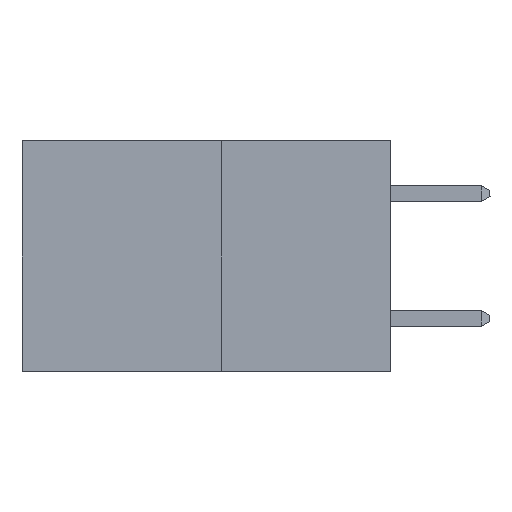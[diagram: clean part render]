
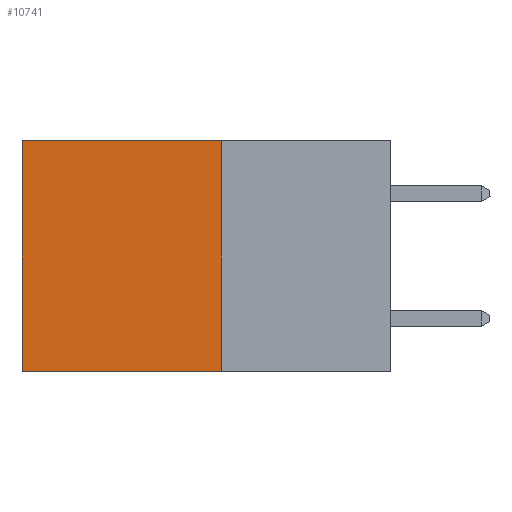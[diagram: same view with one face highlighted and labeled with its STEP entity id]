
A CAD part, left-side view. The second image highlights one B-rep face of the part: STEP entity #10741.
In plain terms, the highlighted planar face has unit normal (-1, 0, 0).
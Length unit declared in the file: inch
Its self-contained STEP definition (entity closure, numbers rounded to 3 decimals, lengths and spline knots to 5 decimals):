
#1203 = VERTEX_POINT ( 'NONE', #9209 ) ;
#1303 = DIRECTION ( 'NONE',  ( 0., 0., -1. ) ) ;
#1723 = VERTEX_POINT ( 'NONE', #7857 ) ;
#1883 = ORIENTED_EDGE ( 'NONE', *, *, #22564, .T. ) ;
#1886 = CARTESIAN_POINT ( 'NONE',  ( 0.277, 0.27, -0.37 ) ) ;
#2969 = EDGE_CURVE ( 'NONE', #15970, #17528, #15374, .T. ) ;
#4008 = FACE_OUTER_BOUND ( 'NONE', #21508, .T. ) ;
#6388 = DIRECTION ( 'NONE',  ( 0., 0., -1. ) ) ;
#6824 = PLANE ( 'NONE',  #8939 ) ;
#6925 = DIRECTION ( 'NONE',  ( 0., 0., -1. ) ) ;
#7279 = VECTOR ( 'NONE', #1303, 39.37008 ) ;
#7857 = CARTESIAN_POINT ( 'NONE',  ( 0.277, 0.59, 0. ) ) ;
#8897 = VECTOR ( 'NONE', #14996, 39.37008 ) ;
#8939 = AXIS2_PLACEMENT_3D ( 'NONE', #13415, #19877, #6925 ) ;
#9209 = CARTESIAN_POINT ( 'NONE',  ( 0.277, 0.59, -0.37 ) ) ;
#9581 = VECTOR ( 'NONE', #6388, 39.37008 ) ;
#10741 = ADVANCED_FACE ( 'NONE', ( #4008 ), #6824, .F. ) ;
#11475 = ORIENTED_EDGE ( 'NONE', *, *, #27936, .F. ) ;
#12158 = ORIENTED_EDGE ( 'NONE', *, *, #2969, .F. ) ;
#13069 = LINE ( 'NONE', #27168, #7279 ) ;
#13316 = LINE ( 'NONE', #1886, #8897 ) ;
#13415 = CARTESIAN_POINT ( 'NONE',  ( 0.277, 0.27, -0.37 ) ) ;
#14996 = DIRECTION ( 'NONE',  ( 0., 1., 0. ) ) ;
#15374 = LINE ( 'NONE', #19117, #9581 ) ;
#15970 = VERTEX_POINT ( 'NONE', #25716 ) ;
#16583 = ORIENTED_EDGE ( 'NONE', *, *, #26253, .T. ) ;
#17528 = VERTEX_POINT ( 'NONE', #22457 ) ;
#19117 = CARTESIAN_POINT ( 'NONE',  ( 0.277, 0.27, -0.37 ) ) ;
#19877 = DIRECTION ( 'NONE',  ( 1., 0., 0. ) ) ;
#21508 = EDGE_LOOP ( 'NONE', ( #16583, #11475, #12158, #1883 ) ) ;
#22233 = CARTESIAN_POINT ( 'NONE',  ( 0.277, 0.27, 0. ) ) ;
#22457 = CARTESIAN_POINT ( 'NONE',  ( 0.277, 0.27, -0.37 ) ) ;
#22564 = EDGE_CURVE ( 'NONE', #15970, #1723, #27939, .T. ) ;
#23663 = VECTOR ( 'NONE', #24382, 39.37008 ) ;
#24382 = DIRECTION ( 'NONE',  ( 0., 1., 0. ) ) ;
#25716 = CARTESIAN_POINT ( 'NONE',  ( 0.277, 0.27, 0. ) ) ;
#26253 = EDGE_CURVE ( 'NONE', #1723, #1203, #13069, .T. ) ;
#27168 = CARTESIAN_POINT ( 'NONE',  ( 0.277, 0.59, -0.37 ) ) ;
#27936 = EDGE_CURVE ( 'NONE', #17528, #1203, #13316, .T. ) ;
#27939 = LINE ( 'NONE', #22233, #23663 ) ;
